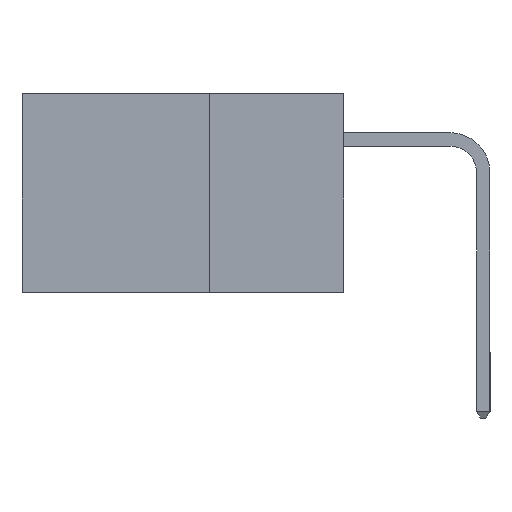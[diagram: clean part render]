
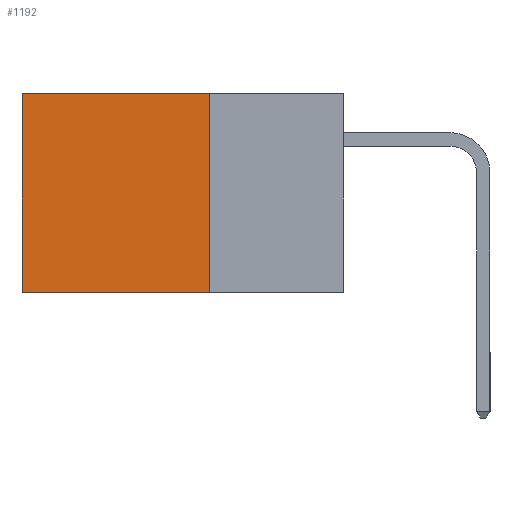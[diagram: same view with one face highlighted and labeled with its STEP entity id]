
A CAD part, left-side view. The second image highlights one B-rep face of the part: STEP entity #1192.
In plain terms, the highlighted planar face has unit normal (-1, 0, 0).
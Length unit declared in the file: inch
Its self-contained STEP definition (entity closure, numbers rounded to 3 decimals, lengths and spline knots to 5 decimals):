
#1192 = ADVANCED_FACE ( 'NONE', ( #5196 ), #2983, .F. ) ;
#1832 = DIRECTION ( 'NONE',  ( 0., 0., -1. ) ) ;
#2025 = LINE ( 'NONE', #10170, #20536 ) ;
#2271 = EDGE_CURVE ( 'NONE', #21555, #19851, #2025, .T. ) ;
#2627 = VERTEX_POINT ( 'NONE', #4737 ) ;
#2983 = PLANE ( 'NONE',  #17906 ) ;
#3023 = DIRECTION ( 'NONE',  ( 1., 0., 0. ) ) ;
#3185 = DIRECTION ( 'NONE',  ( 0., 0., -1. ) ) ;
#3497 = VECTOR ( 'NONE', #1832, 39.37008 ) ;
#3572 = CARTESIAN_POINT ( 'NONE',  ( 0.298, 0.25, 0. ) ) ;
#3600 = LINE ( 'NONE', #21000, #23805 ) ;
#4650 = EDGE_LOOP ( 'NONE', ( #23234, #18754, #9137, #20166 ) ) ;
#4737 = CARTESIAN_POINT ( 'NONE',  ( 0.298, 0.6, -0.37 ) ) ;
#5196 = FACE_OUTER_BOUND ( 'NONE', #4650, .T. ) ;
#9137 = ORIENTED_EDGE ( 'NONE', *, *, #12321, .F. ) ;
#10140 = DIRECTION ( 'NONE',  ( 0., 1., 0. ) ) ;
#10170 = CARTESIAN_POINT ( 'NONE',  ( 0.298, 0.25, 0. ) ) ;
#12321 = EDGE_CURVE ( 'NONE', #21555, #18639, #3600, .T. ) ;
#13081 = EDGE_CURVE ( 'NONE', #18639, #2627, #19486, .T. ) ;
#13962 = VECTOR ( 'NONE', #23684, 39.37008 ) ;
#14387 = CARTESIAN_POINT ( 'NONE',  ( 0.298, 0.6, 0. ) ) ;
#15462 = DIRECTION ( 'NONE',  ( 0., 0., -1. ) ) ;
#16389 = CARTESIAN_POINT ( 'NONE',  ( 0.298, 0.25, -0.37 ) ) ;
#16650 = CARTESIAN_POINT ( 'NONE',  ( 0.298, 0.6, 0. ) ) ;
#17906 = AXIS2_PLACEMENT_3D ( 'NONE', #3572, #3023, #3185 ) ;
#18639 = VERTEX_POINT ( 'NONE', #23468 ) ;
#18754 = ORIENTED_EDGE ( 'NONE', *, *, #13081, .F. ) ;
#19486 = LINE ( 'NONE', #16389, #13962 ) ;
#19851 = VERTEX_POINT ( 'NONE', #14387 ) ;
#20166 = ORIENTED_EDGE ( 'NONE', *, *, #2271, .T. ) ;
#20536 = VECTOR ( 'NONE', #10140, 39.37008 ) ;
#20569 = EDGE_CURVE ( 'NONE', #19851, #2627, #22559, .T. ) ;
#21000 = CARTESIAN_POINT ( 'NONE',  ( 0.298, 0.25, 0. ) ) ;
#21093 = CARTESIAN_POINT ( 'NONE',  ( 0.298, 0.25, 0. ) ) ;
#21555 = VERTEX_POINT ( 'NONE', #21093 ) ;
#22559 = LINE ( 'NONE', #16650, #3497 ) ;
#23234 = ORIENTED_EDGE ( 'NONE', *, *, #20569, .T. ) ;
#23468 = CARTESIAN_POINT ( 'NONE',  ( 0.298, 0.25, -0.37 ) ) ;
#23684 = DIRECTION ( 'NONE',  ( 0., 1., 0. ) ) ;
#23805 = VECTOR ( 'NONE', #15462, 39.37008 ) ;
